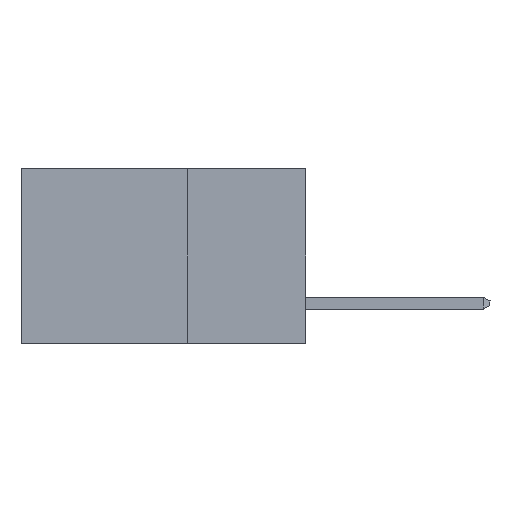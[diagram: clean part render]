
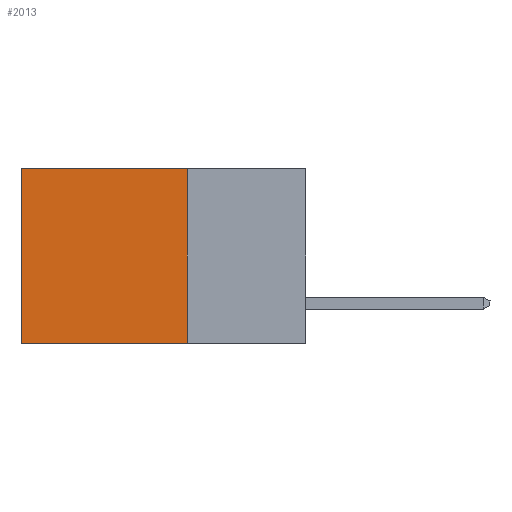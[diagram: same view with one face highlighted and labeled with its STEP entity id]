
A CAD part, left-side view. The second image highlights one B-rep face of the part: STEP entity #2013.
In plain terms, the highlighted planar face has unit normal (-1, 0, 0).
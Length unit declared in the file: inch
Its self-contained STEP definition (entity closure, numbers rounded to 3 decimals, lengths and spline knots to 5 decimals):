
#105 = DIRECTION ( 'NONE',  ( 0., 1., 0. ) ) ;
#374 = CARTESIAN_POINT ( 'NONE',  ( 0.298, 0.6, 0. ) ) ;
#479 = ORIENTED_EDGE ( 'NONE', *, *, #7944, .F. ) ;
#665 = VERTEX_POINT ( 'NONE', #7914 ) ;
#1057 = CARTESIAN_POINT ( 'NONE',  ( 0.298, 0.25, 0. ) ) ;
#1352 = DIRECTION ( 'NONE',  ( 0., 0., -1. ) ) ;
#1374 = EDGE_CURVE ( 'NONE', #4731, #4597, #13644, .T. ) ;
#1962 = CARTESIAN_POINT ( 'NONE',  ( 0.298, 0.25, 0. ) ) ;
#2013 = ADVANCED_FACE ( 'NONE', ( #12256 ), #11697, .F. ) ;
#2376 = CARTESIAN_POINT ( 'NONE',  ( 0.298, 0.25, 0. ) ) ;
#2977 = VECTOR ( 'NONE', #5392, 39.37008 ) ;
#3491 = ORIENTED_EDGE ( 'NONE', *, *, #1374, .F. ) ;
#4090 = CARTESIAN_POINT ( 'NONE',  ( 0.298, 0.6, -0.37 ) ) ;
#4269 = VECTOR ( 'NONE', #4794, 39.37008 ) ;
#4564 = EDGE_CURVE ( 'NONE', #665, #10347, #10861, .T. ) ;
#4597 = VERTEX_POINT ( 'NONE', #13491 ) ;
#4678 = ORIENTED_EDGE ( 'NONE', *, *, #8393, .T. ) ;
#4731 = VERTEX_POINT ( 'NONE', #1057 ) ;
#4794 = DIRECTION ( 'NONE',  ( 0., 0., -1. ) ) ;
#5392 = DIRECTION ( 'NONE',  ( 0., 1., 0. ) ) ;
#7448 = EDGE_LOOP ( 'NONE', ( #7762, #479, #3491, #4678 ) ) ;
#7679 = LINE ( 'NONE', #2376, #11081 ) ;
#7762 = ORIENTED_EDGE ( 'NONE', *, *, #4564, .T. ) ;
#7914 = CARTESIAN_POINT ( 'NONE',  ( 0.298, 0.6, 0. ) ) ;
#7944 = EDGE_CURVE ( 'NONE', #4597, #10347, #13131, .T. ) ;
#8045 = VECTOR ( 'NONE', #1352, 39.37008 ) ;
#8393 = EDGE_CURVE ( 'NONE', #4731, #665, #7679, .T. ) ;
#8499 = CARTESIAN_POINT ( 'NONE',  ( 0.298, 0.25, -0.37 ) ) ;
#8750 = AXIS2_PLACEMENT_3D ( 'NONE', #1962, #9606, #12926 ) ;
#9606 = DIRECTION ( 'NONE',  ( 1., 0., 0. ) ) ;
#10347 = VERTEX_POINT ( 'NONE', #4090 ) ;
#10861 = LINE ( 'NONE', #374, #4269 ) ;
#11081 = VECTOR ( 'NONE', #105, 39.37008 ) ;
#11697 = PLANE ( 'NONE',  #8750 ) ;
#12256 = FACE_OUTER_BOUND ( 'NONE', #7448, .T. ) ;
#12926 = DIRECTION ( 'NONE',  ( 0., 0., -1. ) ) ;
#13131 = LINE ( 'NONE', #8499, #2977 ) ;
#13233 = CARTESIAN_POINT ( 'NONE',  ( 0.298, 0.25, 0. ) ) ;
#13491 = CARTESIAN_POINT ( 'NONE',  ( 0.298, 0.25, -0.37 ) ) ;
#13644 = LINE ( 'NONE', #13233, #8045 ) ;
